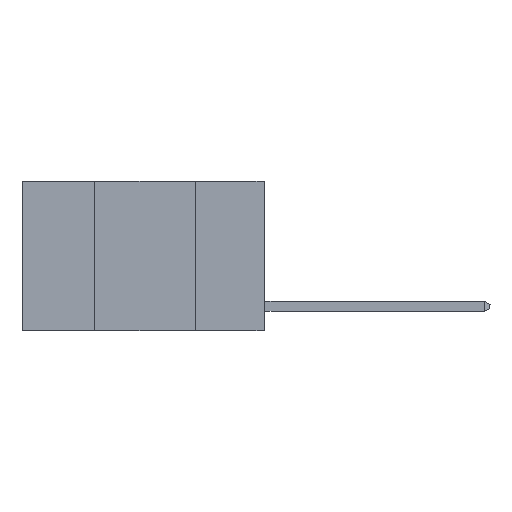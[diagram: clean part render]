
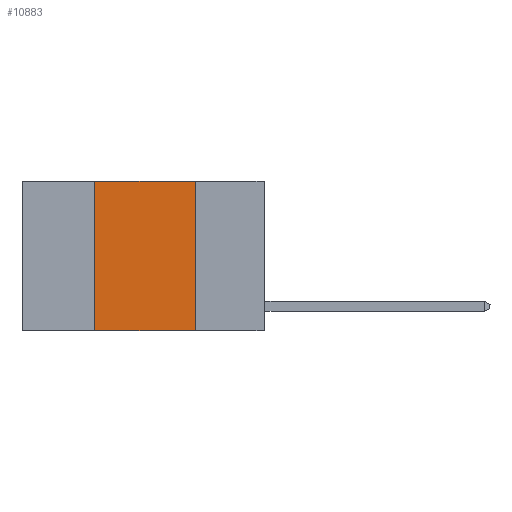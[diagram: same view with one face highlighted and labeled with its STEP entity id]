
A CAD part, left-side view. The second image highlights one B-rep face of the part: STEP entity #10883.
In plain terms, the highlighted planar face has unit normal (-1, 0, 0).
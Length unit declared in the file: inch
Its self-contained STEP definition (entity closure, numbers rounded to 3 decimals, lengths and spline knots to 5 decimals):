
#38 = EDGE_CURVE ( 'NONE', #11302, #8879, #3470, .T. ) ;
#312 = DIRECTION ( 'NONE',  ( 0., 0., 1. ) ) ;
#381 = DIRECTION ( 'NONE',  ( 0., 0., -1. ) ) ;
#779 = CARTESIAN_POINT ( 'NONE',  ( 0., 0.17, -0.37 ) ) ;
#837 = VECTOR ( 'NONE', #3309, 39.37008 ) ;
#954 = CARTESIAN_POINT ( 'NONE',  ( 0., 0.17, 0. ) ) ;
#1134 = LINE ( 'NONE', #3070, #7427 ) ;
#1926 = CARTESIAN_POINT ( 'NONE',  ( 0., 0.17, 0. ) ) ;
#2072 = CARTESIAN_POINT ( 'NONE',  ( 0., 0.42, 0. ) ) ;
#3067 = LINE ( 'NONE', #8401, #837 ) ;
#3070 = CARTESIAN_POINT ( 'NONE',  ( 0., 0.6, -0.37 ) ) ;
#3137 = EDGE_CURVE ( 'NONE', #5527, #6226, #6875, .T. ) ;
#3309 = DIRECTION ( 'NONE',  ( 0., -1., 0. ) ) ;
#3470 = LINE ( 'NONE', #954, #4584 ) ;
#3914 = DIRECTION ( 'NONE',  ( 1., 0., 0. ) ) ;
#4584 = VECTOR ( 'NONE', #7392, 39.37008 ) ;
#5460 = VECTOR ( 'NONE', #312, 39.37008 ) ;
#5501 = EDGE_LOOP ( 'NONE', ( #11593, #7970, #5975, #6928 ) ) ;
#5527 = VERTEX_POINT ( 'NONE', #8822 ) ;
#5975 = ORIENTED_EDGE ( 'NONE', *, *, #3137, .F. ) ;
#6226 = VERTEX_POINT ( 'NONE', #10932 ) ;
#6875 = LINE ( 'NONE', #2072, #5460 ) ;
#6928 = ORIENTED_EDGE ( 'NONE', *, *, #9128, .T. ) ;
#7392 = DIRECTION ( 'NONE',  ( 0., 0., -1. ) ) ;
#7427 = VECTOR ( 'NONE', #10287, 39.37008 ) ;
#7437 = AXIS2_PLACEMENT_3D ( 'NONE', #11160, #3914, #381 ) ;
#7970 = ORIENTED_EDGE ( 'NONE', *, *, #10279, .F. ) ;
#8401 = CARTESIAN_POINT ( 'NONE',  ( 0., 0.6, 0. ) ) ;
#8822 = CARTESIAN_POINT ( 'NONE',  ( 0., 0.42, -0.37 ) ) ;
#8879 = VERTEX_POINT ( 'NONE', #779 ) ;
#9128 = EDGE_CURVE ( 'NONE', #5527, #8879, #1134, .T. ) ;
#9477 = PLANE ( 'NONE',  #7437 ) ;
#10279 = EDGE_CURVE ( 'NONE', #6226, #11302, #3067, .T. ) ;
#10287 = DIRECTION ( 'NONE',  ( 0., -1., 0. ) ) ;
#10883 = ADVANCED_FACE ( 'NONE', ( #11347 ), #9477, .F. ) ;
#10932 = CARTESIAN_POINT ( 'NONE',  ( 0., 0.42, 0. ) ) ;
#11160 = CARTESIAN_POINT ( 'NONE',  ( 0., 0.6, 0. ) ) ;
#11302 = VERTEX_POINT ( 'NONE', #1926 ) ;
#11347 = FACE_OUTER_BOUND ( 'NONE', #5501, .T. ) ;
#11593 = ORIENTED_EDGE ( 'NONE', *, *, #38, .F. ) ;
